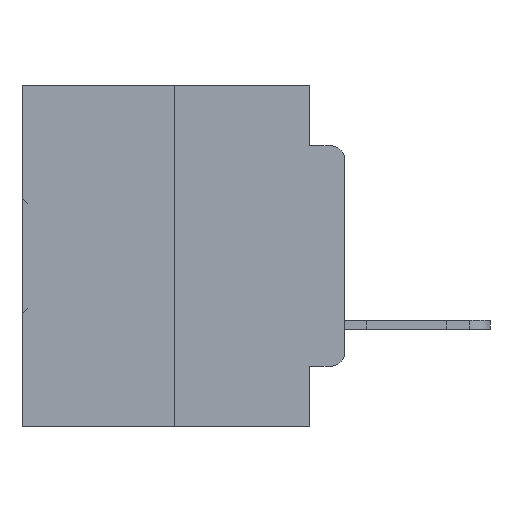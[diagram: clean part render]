
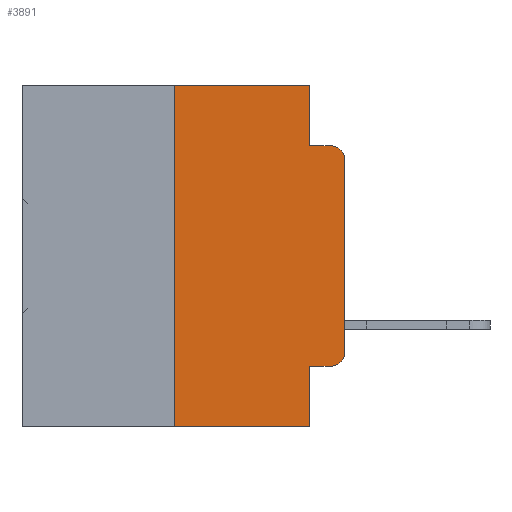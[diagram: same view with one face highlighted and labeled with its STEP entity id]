
A CAD part, left-side view. The second image highlights one B-rep face of the part: STEP entity #3891.
In plain terms, the highlighted planar face has unit normal (-1, 0, 0).
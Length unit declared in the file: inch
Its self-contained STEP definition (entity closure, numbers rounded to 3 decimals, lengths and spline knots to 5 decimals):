
#229 = CARTESIAN_POINT ( 'NONE',  ( 0., 0.051, -0.4115 ) ) ;
#468 = LINE ( 'NONE', #33178, #7115 ) ;
#537 = ORIENTED_EDGE ( 'NONE', *, *, #19938, .T. ) ;
#572 = EDGE_LOOP ( 'NONE', ( #22712, #11526, #33247, #13250, #21419, #1875, #26610, #20122, #14568, #537 ) ) ;
#652 = CARTESIAN_POINT ( 'NONE',  ( 0., 0.051, 0. ) ) ;
#850 = DIRECTION ( 'NONE',  ( 0., 0., 1. ) ) ;
#1875 = ORIENTED_EDGE ( 'NONE', *, *, #15124, .F. ) ;
#1960 = CARTESIAN_POINT ( 'NONE',  ( 0., 0.02, -0.4115 ) ) ;
#3075 = DIRECTION ( 'NONE',  ( 0., 0., 1. ) ) ;
#3512 = DIRECTION ( 'NONE',  ( 0., 0., -1. ) ) ;
#3826 = VECTOR ( 'NONE', #13182, 39.37008 ) ;
#3891 = ADVANCED_FACE ( 'NONE', ( #20336 ), #6017, .F. ) ;
#4427 = DIRECTION ( 'NONE',  ( -1., 0., 0. ) ) ;
#5031 = VECTOR ( 'NONE', #10908, 39.37008 ) ;
#5064 = VECTOR ( 'NONE', #20580, 39.37008 ) ;
#5807 = EDGE_CURVE ( 'NONE', #9344, #24766, #19756, .T. ) ;
#6006 = AXIS2_PLACEMENT_3D ( 'NONE', #28229, #29030, #3512 ) ;
#6017 = PLANE ( 'NONE',  #6006 ) ;
#6485 = LINE ( 'NONE', #33790, #35507 ) ;
#6490 = DIRECTION ( 'NONE',  ( 0., -1., 0. ) ) ;
#7115 = VECTOR ( 'NONE', #3075, 39.37008 ) ;
#8785 = CARTESIAN_POINT ( 'NONE',  ( 0., 0.051, -0.5 ) ) ;
#9185 = CARTESIAN_POINT ( 'NONE',  ( 0., 0.051, -0.0885 ) ) ;
#9344 = VERTEX_POINT ( 'NONE', #652 ) ;
#10226 = EDGE_CURVE ( 'NONE', #16915, #14390, #19789, .T. ) ;
#10605 = CARTESIAN_POINT ( 'NONE',  ( 0., 0.051, 0. ) ) ;
#10908 = DIRECTION ( 'NONE',  ( 0., 0., -1. ) ) ;
#11526 = ORIENTED_EDGE ( 'NONE', *, *, #21332, .T. ) ;
#12134 = EDGE_CURVE ( 'NONE', #21522, #28007, #468, .T. ) ;
#13182 = DIRECTION ( 'NONE',  ( 0., -1., 0. ) ) ;
#13250 = ORIENTED_EDGE ( 'NONE', *, *, #5807, .F. ) ;
#13275 = VECTOR ( 'NONE', #6490, 39.37008 ) ;
#13832 = CARTESIAN_POINT ( 'NONE',  ( 0., 0.02, -0.1085 ) ) ;
#14390 = VERTEX_POINT ( 'NONE', #8785 ) ;
#14568 = ORIENTED_EDGE ( 'NONE', *, *, #33334, .T. ) ;
#14808 = CARTESIAN_POINT ( 'NONE',  ( 0., 0.25, -0.5 ) ) ;
#14827 = VERTEX_POINT ( 'NONE', #16269 ) ;
#15124 = EDGE_CURVE ( 'NONE', #16915, #33772, #6485, .T. ) ;
#16269 = CARTESIAN_POINT ( 'NONE',  ( 0., 0.02, -0.0885 ) ) ;
#16617 = DIRECTION ( 'NONE',  ( 0., 0., -1. ) ) ;
#16681 = VERTEX_POINT ( 'NONE', #35429 ) ;
#16915 = VERTEX_POINT ( 'NONE', #14808 ) ;
#16958 = DIRECTION ( 'NONE',  ( 0., -1., 0. ) ) ;
#17764 = EDGE_CURVE ( 'NONE', #33772, #9344, #18574, .T. ) ;
#17830 = CARTESIAN_POINT ( 'NONE',  ( 0., 0., -0.1085 ) ) ;
#18574 = LINE ( 'NONE', #29618, #3826 ) ;
#18803 = EDGE_CURVE ( 'NONE', #16681, #14390, #34984, .T. ) ;
#19576 = VECTOR ( 'NONE', #16958, 39.37008 ) ;
#19756 = LINE ( 'NONE', #10605, #5031 ) ;
#19789 = LINE ( 'NONE', #20947, #5064 ) ;
#19938 = EDGE_CURVE ( 'NONE', #33704, #21522, #26227, .T. ) ;
#20122 = ORIENTED_EDGE ( 'NONE', *, *, #18803, .F. ) ;
#20128 = CARTESIAN_POINT ( 'NONE',  ( 0., 0.051, -0.0885 ) ) ;
#20336 = FACE_OUTER_BOUND ( 'NONE', #572, .T. ) ;
#20421 = LINE ( 'NONE', #229, #19576 ) ;
#20580 = DIRECTION ( 'NONE',  ( 0., -1., 0. ) ) ;
#20794 = CARTESIAN_POINT ( 'NONE',  ( 0., 0.051, 0. ) ) ;
#20947 = CARTESIAN_POINT ( 'NONE',  ( 0., 0.473, -0.5 ) ) ;
#21010 = CARTESIAN_POINT ( 'NONE',  ( 0., 0.02, -0.3915 ) ) ;
#21332 = EDGE_CURVE ( 'NONE', #28007, #14827, #25298, .T. ) ;
#21419 = ORIENTED_EDGE ( 'NONE', *, *, #17764, .F. ) ;
#21522 = VERTEX_POINT ( 'NONE', #25647 ) ;
#22712 = ORIENTED_EDGE ( 'NONE', *, *, #12134, .T. ) ;
#23615 = DIRECTION ( 'NONE',  ( 0., 0., -1. ) ) ;
#23824 = DIRECTION ( 'NONE',  ( 0., 0., -1. ) ) ;
#24766 = VERTEX_POINT ( 'NONE', #20128 ) ;
#25298 = CIRCLE ( 'NONE', #33445, 0.02 ) ;
#25647 = CARTESIAN_POINT ( 'NONE',  ( 0., 0., -0.3915 ) ) ;
#26065 = AXIS2_PLACEMENT_3D ( 'NONE', #21010, #4427, #23824 ) ;
#26227 = CIRCLE ( 'NONE', #26065, 0.02 ) ;
#26610 = ORIENTED_EDGE ( 'NONE', *, *, #10226, .T. ) ;
#27088 = VECTOR ( 'NONE', #23615, 39.37008 ) ;
#28007 = VERTEX_POINT ( 'NONE', #17830 ) ;
#28229 = CARTESIAN_POINT ( 'NONE',  ( 0., 0.473, 0. ) ) ;
#29030 = DIRECTION ( 'NONE',  ( 1., 0., 0. ) ) ;
#29618 = CARTESIAN_POINT ( 'NONE',  ( 0., 0.473, 0. ) ) ;
#30478 = EDGE_CURVE ( 'NONE', #24766, #14827, #34926, .T. ) ;
#32500 = CARTESIAN_POINT ( 'NONE',  ( 0., 0.25, 0. ) ) ;
#32851 = DIRECTION ( 'NONE',  ( -1., 0., 0. ) ) ;
#33178 = CARTESIAN_POINT ( 'NONE',  ( 0., 0., 0. ) ) ;
#33247 = ORIENTED_EDGE ( 'NONE', *, *, #30478, .F. ) ;
#33334 = EDGE_CURVE ( 'NONE', #16681, #33704, #20421, .T. ) ;
#33445 = AXIS2_PLACEMENT_3D ( 'NONE', #13832, #32851, #16617 ) ;
#33704 = VERTEX_POINT ( 'NONE', #1960 ) ;
#33772 = VERTEX_POINT ( 'NONE', #32500 ) ;
#33790 = CARTESIAN_POINT ( 'NONE',  ( 0., 0.25, 0. ) ) ;
#34926 = LINE ( 'NONE', #9185, #13275 ) ;
#34984 = LINE ( 'NONE', #20794, #27088 ) ;
#35429 = CARTESIAN_POINT ( 'NONE',  ( 0., 0.051, -0.4115 ) ) ;
#35507 = VECTOR ( 'NONE', #850, 39.37008 ) ;
